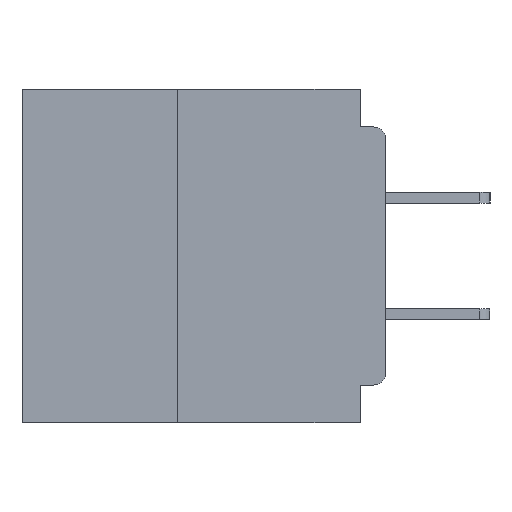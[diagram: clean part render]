
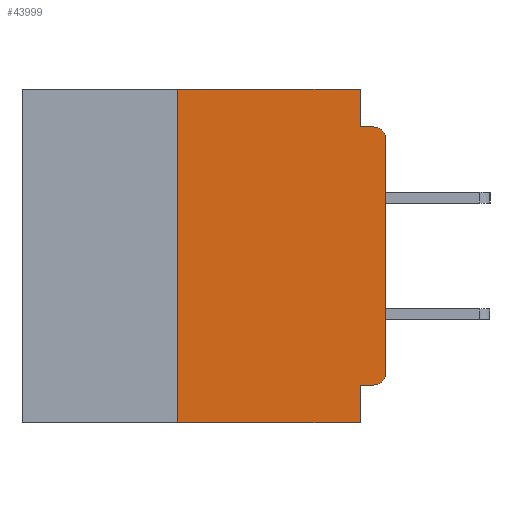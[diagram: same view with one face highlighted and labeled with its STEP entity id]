
A CAD part, left-side view. The second image highlights one B-rep face of the part: STEP entity #43999.
In plain terms, the highlighted planar face has unit normal (-1, 0, 0).
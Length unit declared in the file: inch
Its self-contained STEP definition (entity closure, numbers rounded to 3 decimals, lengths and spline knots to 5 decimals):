
#71 = FACE_OUTER_BOUND ( 'NONE', #48109, .T. ) ;
#743 = EDGE_CURVE ( 'NONE', #30374, #35759, #6260, .T. ) ;
#1629 = VERTEX_POINT ( 'NONE', #19487 ) ;
#1870 = CARTESIAN_POINT ( 'NONE',  ( 0., 0.031, -0.045 ) ) ;
#2711 = LINE ( 'NONE', #12236, #23395 ) ;
#4293 = DIRECTION ( 'NONE',  ( 0., -1., 0. ) ) ;
#4589 = CARTESIAN_POINT ( 'NONE',  ( 0., 0., -0.355 ) ) ;
#5313 = EDGE_CURVE ( 'NONE', #33596, #18801, #17130, .T. ) ;
#5609 = DIRECTION ( 'NONE',  ( -1., 0., 0. ) ) ;
#6260 = LINE ( 'NONE', #32178, #36094 ) ;
#6570 = DIRECTION ( 'NONE',  ( 1., 0., 0. ) ) ;
#6839 = CARTESIAN_POINT ( 'NONE',  ( 0., 0.031, -0.4 ) ) ;
#8176 = LINE ( 'NONE', #42889, #27658 ) ;
#8516 = DIRECTION ( 'NONE',  ( 0., -1., 0. ) ) ;
#10243 = EDGE_CURVE ( 'NONE', #33596, #42770, #20557, .T. ) ;
#11164 = CARTESIAN_POINT ( 'NONE',  ( 0., 0.25, -0.4 ) ) ;
#11236 = CIRCLE ( 'NONE', #29329, 0.015 ) ;
#11561 = DIRECTION ( 'NONE',  ( 0., 0., 1. ) ) ;
#12236 = CARTESIAN_POINT ( 'NONE',  ( 0., 0., -0.045 ) ) ;
#12462 = LINE ( 'NONE', #41294, #22793 ) ;
#12652 = DIRECTION ( 'NONE',  ( 0., -1., 0. ) ) ;
#13561 = ORIENTED_EDGE ( 'NONE', *, *, #10243, .F. ) ;
#15617 = DIRECTION ( 'NONE',  ( 0., 0., -1. ) ) ;
#15901 = LINE ( 'NONE', #38729, #27499 ) ;
#17001 = DIRECTION ( 'NONE',  ( 0., 0., -1. ) ) ;
#17029 = ORIENTED_EDGE ( 'NONE', *, *, #32502, .T. ) ;
#17082 = ORIENTED_EDGE ( 'NONE', *, *, #18290, .F. ) ;
#17105 = DIRECTION ( 'NONE',  ( -1., 0., 0. ) ) ;
#17130 = CIRCLE ( 'NONE', #42983, 0.015 ) ;
#17321 = CARTESIAN_POINT ( 'NONE',  ( 0., 0.015, -0.34 ) ) ;
#17653 = LINE ( 'NONE', #11164, #38295 ) ;
#17860 = ORIENTED_EDGE ( 'NONE', *, *, #40792, .T. ) ;
#18126 = CARTESIAN_POINT ( 'NONE',  ( 0., 0.437, 0. ) ) ;
#18290 = EDGE_CURVE ( 'NONE', #42770, #35759, #12462, .T. ) ;
#18766 = VERTEX_POINT ( 'NONE', #1870 ) ;
#18801 = VERTEX_POINT ( 'NONE', #36885 ) ;
#18980 = DIRECTION ( 'NONE',  ( 0., 0., 1. ) ) ;
#19487 = CARTESIAN_POINT ( 'NONE',  ( 0., 0.25, 0. ) ) ;
#19895 = CARTESIAN_POINT ( 'NONE',  ( 0., 0.031, 0. ) ) ;
#20130 = ORIENTED_EDGE ( 'NONE', *, *, #48224, .F. ) ;
#20557 = LINE ( 'NONE', #4589, #49654 ) ;
#20601 = EDGE_CURVE ( 'NONE', #1629, #36008, #30509, .T. ) ;
#20984 = VERTEX_POINT ( 'NONE', #46511 ) ;
#20986 = VERTEX_POINT ( 'NONE', #31216 ) ;
#22793 = VECTOR ( 'NONE', #29831, 39.37008 ) ;
#23395 = VECTOR ( 'NONE', #8516, 39.37008 ) ;
#27499 = VECTOR ( 'NONE', #11561, 39.37008 ) ;
#27658 = VECTOR ( 'NONE', #15617, 39.37008 ) ;
#27797 = ORIENTED_EDGE ( 'NONE', *, *, #33102, .F. ) ;
#28957 = CARTESIAN_POINT ( 'NONE',  ( 0., 0.015, -0.06 ) ) ;
#29329 = AXIS2_PLACEMENT_3D ( 'NONE', #28957, #5609, #32880 ) ;
#29831 = DIRECTION ( 'NONE',  ( 0., 0., -1. ) ) ;
#29880 = PLANE ( 'NONE',  #43632 ) ;
#30374 = VERTEX_POINT ( 'NONE', #47192 ) ;
#30469 = CARTESIAN_POINT ( 'NONE',  ( 0., 0.031, -0.355 ) ) ;
#30509 = LINE ( 'NONE', #44338, #49742 ) ;
#31216 = CARTESIAN_POINT ( 'NONE',  ( 0., 0., -0.06 ) ) ;
#32178 = CARTESIAN_POINT ( 'NONE',  ( 0., 0.437, -0.4 ) ) ;
#32502 = EDGE_CURVE ( 'NONE', #18801, #20986, #15901, .T. ) ;
#32880 = DIRECTION ( 'NONE',  ( 0., 0., -1. ) ) ;
#33102 = EDGE_CURVE ( 'NONE', #30374, #1629, #17653, .T. ) ;
#33596 = VERTEX_POINT ( 'NONE', #41832 ) ;
#33821 = DIRECTION ( 'NONE',  ( 0., 0., -1. ) ) ;
#35736 = DIRECTION ( 'NONE',  ( 0., 1., 0. ) ) ;
#35759 = VERTEX_POINT ( 'NONE', #6839 ) ;
#36008 = VERTEX_POINT ( 'NONE', #19895 ) ;
#36094 = VECTOR ( 'NONE', #4293, 39.37008 ) ;
#36626 = EDGE_CURVE ( 'NONE', #36008, #18766, #8176, .T. ) ;
#36885 = CARTESIAN_POINT ( 'NONE',  ( 0., 0., -0.34 ) ) ;
#38295 = VECTOR ( 'NONE', #18980, 39.37008 ) ;
#38729 = CARTESIAN_POINT ( 'NONE',  ( 0., 0., 0. ) ) ;
#40792 = EDGE_CURVE ( 'NONE', #20986, #20984, #11236, .T. ) ;
#41294 = CARTESIAN_POINT ( 'NONE',  ( 0., 0.031, -0.4 ) ) ;
#41832 = CARTESIAN_POINT ( 'NONE',  ( 0., 0.015, -0.355 ) ) ;
#42658 = ORIENTED_EDGE ( 'NONE', *, *, #5313, .T. ) ;
#42770 = VERTEX_POINT ( 'NONE', #30469 ) ;
#42889 = CARTESIAN_POINT ( 'NONE',  ( 0., 0.031, 0. ) ) ;
#42983 = AXIS2_PLACEMENT_3D ( 'NONE', #17321, #17105, #17001 ) ;
#43054 = ORIENTED_EDGE ( 'NONE', *, *, #36626, .F. ) ;
#43632 = AXIS2_PLACEMENT_3D ( 'NONE', #18126, #6570, #33821 ) ;
#43999 = ADVANCED_FACE ( 'NONE', ( #71 ), #29880, .F. ) ;
#44338 = CARTESIAN_POINT ( 'NONE',  ( 0., 0.437, 0. ) ) ;
#45149 = ORIENTED_EDGE ( 'NONE', *, *, #20601, .F. ) ;
#46511 = CARTESIAN_POINT ( 'NONE',  ( 0., 0.015, -0.045 ) ) ;
#47192 = CARTESIAN_POINT ( 'NONE',  ( 0., 0.25, -0.4 ) ) ;
#48109 = EDGE_LOOP ( 'NONE', ( #17029, #17860, #20130, #43054, #45149, #27797, #49851, #17082, #13561, #42658 ) ) ;
#48224 = EDGE_CURVE ( 'NONE', #18766, #20984, #2711, .T. ) ;
#49654 = VECTOR ( 'NONE', #35736, 39.37008 ) ;
#49742 = VECTOR ( 'NONE', #12652, 39.37008 ) ;
#49851 = ORIENTED_EDGE ( 'NONE', *, *, #743, .T. ) ;
